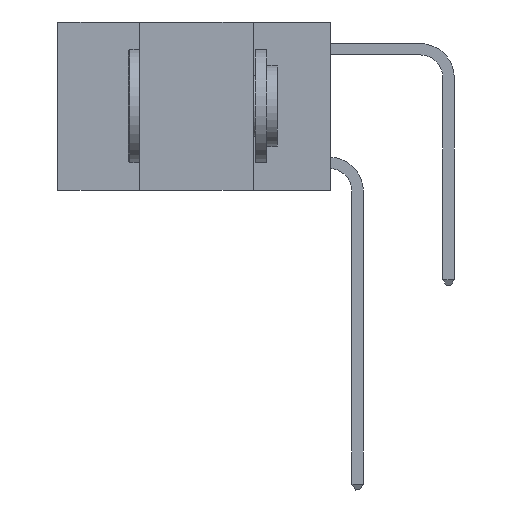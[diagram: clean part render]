
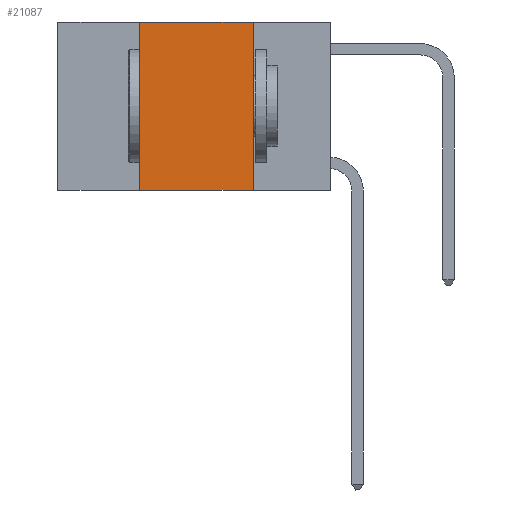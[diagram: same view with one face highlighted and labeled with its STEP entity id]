
A CAD part, left-side view. The second image highlights one B-rep face of the part: STEP entity #21087.
In plain terms, the highlighted planar face has unit normal (-1, 0, 0).
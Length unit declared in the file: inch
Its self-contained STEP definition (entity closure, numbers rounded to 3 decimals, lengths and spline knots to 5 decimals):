
#343 = CARTESIAN_POINT ( 'NONE',  ( 0., 0.42, 0. ) ) ;
#588 = CARTESIAN_POINT ( 'NONE',  ( 0., 0.6, 0. ) ) ;
#1052 = VERTEX_POINT ( 'NONE', #21800 ) ;
#1718 = LINE ( 'NONE', #5410, #6467 ) ;
#1751 = CARTESIAN_POINT ( 'NONE',  ( 0., 0.42, -0.37 ) ) ;
#2054 = VECTOR ( 'NONE', #15650, 39.37008 ) ;
#3680 = CARTESIAN_POINT ( 'NONE',  ( 0., 0.17, 0. ) ) ;
#3787 = LINE ( 'NONE', #343, #10162 ) ;
#5410 = CARTESIAN_POINT ( 'NONE',  ( 0., 0.17, 0. ) ) ;
#5554 = CARTESIAN_POINT ( 'NONE',  ( 0., 0.42, 0. ) ) ;
#5632 = CARTESIAN_POINT ( 'NONE',  ( 0., 0.6, -0.37 ) ) ;
#6467 = VECTOR ( 'NONE', #11954, 39.37008 ) ;
#7359 = DIRECTION ( 'NONE',  ( 0., 0., 1. ) ) ;
#7994 = LINE ( 'NONE', #22198, #12743 ) ;
#9564 = PLANE ( 'NONE',  #14884 ) ;
#9651 = ORIENTED_EDGE ( 'NONE', *, *, #21643, .F. ) ;
#10162 = VECTOR ( 'NONE', #7359, 39.37008 ) ;
#11954 = DIRECTION ( 'NONE',  ( 0., 0., -1. ) ) ;
#12743 = VECTOR ( 'NONE', #13389, 39.37008 ) ;
#12785 = DIRECTION ( 'NONE',  ( 0., 0., -1. ) ) ;
#13126 = VERTEX_POINT ( 'NONE', #5554 ) ;
#13389 = DIRECTION ( 'NONE',  ( 0., -1., 0. ) ) ;
#14007 = VERTEX_POINT ( 'NONE', #1751 ) ;
#14292 = ORIENTED_EDGE ( 'NONE', *, *, #15847, .T. ) ;
#14542 = VERTEX_POINT ( 'NONE', #3680 ) ;
#14838 = FACE_OUTER_BOUND ( 'NONE', #15560, .T. ) ;
#14884 = AXIS2_PLACEMENT_3D ( 'NONE', #588, #21598, #12785 ) ;
#15560 = EDGE_LOOP ( 'NONE', ( #20959, #18663, #9651, #14292 ) ) ;
#15650 = DIRECTION ( 'NONE',  ( 0., -1., 0. ) ) ;
#15847 = EDGE_CURVE ( 'NONE', #14007, #1052, #21237, .T. ) ;
#18663 = ORIENTED_EDGE ( 'NONE', *, *, #22343, .F. ) ;
#20959 = ORIENTED_EDGE ( 'NONE', *, *, #21390, .F. ) ;
#21087 = ADVANCED_FACE ( 'NONE', ( #14838 ), #9564, .F. ) ;
#21237 = LINE ( 'NONE', #5632, #2054 ) ;
#21390 = EDGE_CURVE ( 'NONE', #14542, #1052, #1718, .T. ) ;
#21598 = DIRECTION ( 'NONE',  ( 1., 0., 0. ) ) ;
#21643 = EDGE_CURVE ( 'NONE', #14007, #13126, #3787, .T. ) ;
#21800 = CARTESIAN_POINT ( 'NONE',  ( 0., 0.17, -0.37 ) ) ;
#22198 = CARTESIAN_POINT ( 'NONE',  ( 0., 0.6, 0. ) ) ;
#22343 = EDGE_CURVE ( 'NONE', #13126, #14542, #7994, .T. ) ;
